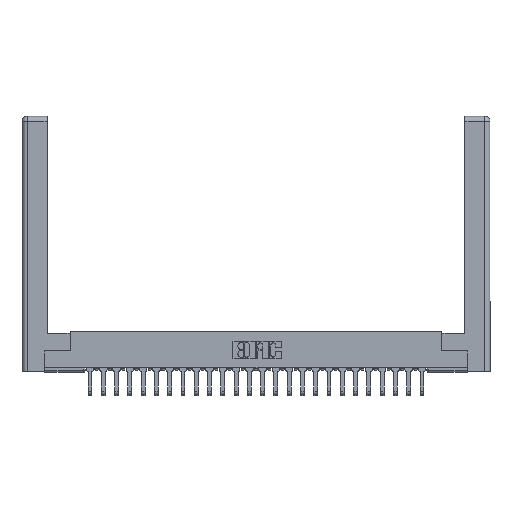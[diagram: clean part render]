
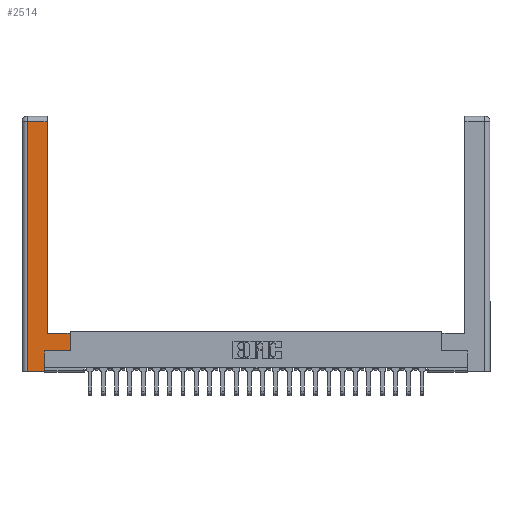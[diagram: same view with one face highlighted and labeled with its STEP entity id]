
A CAD part, top view. The second image highlights one B-rep face of the part: STEP entity #2514.
In plain terms, the highlighted planar face has unit normal (0, 0, 1).
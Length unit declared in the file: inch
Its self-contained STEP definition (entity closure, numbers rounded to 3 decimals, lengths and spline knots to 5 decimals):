
#30 = VECTOR ( 'NONE', #3883, 39.37008 ) ;
#314 = DIRECTION ( 'NONE',  ( -1., 0., 0. ) ) ;
#510 = PLANE ( 'NONE',  #3973 ) ;
#860 = LINE ( 'NONE', #26434, #21745 ) ;
#916 = CARTESIAN_POINT ( 'NONE',  ( 0.565, 0.245, 0. ) ) ;
#1131 = CARTESIAN_POINT ( 'NONE',  ( 0.265, 0.245, 0. ) ) ;
#1563 = CARTESIAN_POINT ( 'NONE',  ( 0.0615, 0., 0. ) ) ;
#1761 = EDGE_CURVE ( 'NONE', #10073, #13633, #22837, .T. ) ;
#2514 = ADVANCED_FACE ( 'NONE', ( #8100 ), #510, .F. ) ;
#2621 = VERTEX_POINT ( 'NONE', #7193 ) ;
#3883 = DIRECTION ( 'NONE',  ( -1., 0., 0. ) ) ;
#3973 = AXIS2_PLACEMENT_3D ( 'NONE', #10960, #25379, #314 ) ;
#4400 = CARTESIAN_POINT ( 'NONE',  ( 0.0615, 0., 0. ) ) ;
#4638 = VERTEX_POINT ( 'NONE', #9826 ) ;
#4655 = VERTEX_POINT ( 'NONE', #23874 ) ;
#4863 = ORIENTED_EDGE ( 'NONE', *, *, #17424, .T. ) ;
#5001 = ORIENTED_EDGE ( 'NONE', *, *, #16443, .T. ) ;
#5208 = DIRECTION ( 'NONE',  ( 0., 1., 0. ) ) ;
#6416 = EDGE_CURVE ( 'NONE', #17836, #2621, #860, .T. ) ;
#7193 = CARTESIAN_POINT ( 'NONE',  ( 0.265, 0., 0. ) ) ;
#7427 = VECTOR ( 'NONE', #21174, 39.37008 ) ;
#7670 = LINE ( 'NONE', #20592, #7977 ) ;
#7977 = VECTOR ( 'NONE', #26803, 39.37008 ) ;
#8100 = FACE_OUTER_BOUND ( 'NONE', #12183, .T. ) ;
#8165 = EDGE_CURVE ( 'NONE', #4655, #4638, #8210, .T. ) ;
#8210 = LINE ( 'NONE', #916, #10479 ) ;
#8674 = CARTESIAN_POINT ( 'NONE',  ( 0.295, 0.45, 0. ) ) ;
#9826 = CARTESIAN_POINT ( 'NONE',  ( 0.565, 0.245, 0. ) ) ;
#10073 = VERTEX_POINT ( 'NONE', #17675 ) ;
#10460 = ORIENTED_EDGE ( 'NONE', *, *, #8165, .T. ) ;
#10479 = VECTOR ( 'NONE', #11371, 39.37008 ) ;
#10960 = CARTESIAN_POINT ( 'NONE',  ( 0., 0., 0. ) ) ;
#11371 = DIRECTION ( 'NONE',  ( 1., 0., 0. ) ) ;
#11389 = ORIENTED_EDGE ( 'NONE', *, *, #15886, .T. ) ;
#11868 = CARTESIAN_POINT ( 'NONE',  ( 0.565, 0.45, 0. ) ) ;
#11870 = VERTEX_POINT ( 'NONE', #26279 ) ;
#12183 = EDGE_LOOP ( 'NONE', ( #4863, #5001, #13068, #23811, #22611, #10460, #11389, #23444 ) ) ;
#12727 = CARTESIAN_POINT ( 'NONE',  ( 0.0615, 2.94, 0. ) ) ;
#13068 = ORIENTED_EDGE ( 'NONE', *, *, #19229, .T. ) ;
#13633 = VERTEX_POINT ( 'NONE', #8674 ) ;
#13782 = LINE ( 'NONE', #1131, #24239 ) ;
#15236 = LINE ( 'NONE', #4400, #7427 ) ;
#15886 = EDGE_CURVE ( 'NONE', #4638, #10073, #22467, .T. ) ;
#16443 = EDGE_CURVE ( 'NONE', #24471, #11870, #17526, .T. ) ;
#17231 = VECTOR ( 'NONE', #26455, 39.37008 ) ;
#17424 = EDGE_CURVE ( 'NONE', #13633, #24471, #7670, .T. ) ;
#17526 = LINE ( 'NONE', #12727, #23720 ) ;
#17675 = CARTESIAN_POINT ( 'NONE',  ( 0.565, 0.45, 0. ) ) ;
#17836 = VERTEX_POINT ( 'NONE', #1563 ) ;
#18246 = CARTESIAN_POINT ( 'NONE',  ( 0.295, 2.94, 0. ) ) ;
#18678 = CARTESIAN_POINT ( 'NONE',  ( 0.295, 0.45, 0. ) ) ;
#19229 = EDGE_CURVE ( 'NONE', #11870, #17836, #15236, .T. ) ;
#20037 = DIRECTION ( 'NONE',  ( 1., 0., 0. ) ) ;
#20592 = CARTESIAN_POINT ( 'NONE',  ( 0.295, 3., 0. ) ) ;
#21174 = DIRECTION ( 'NONE',  ( 0., -1., 0. ) ) ;
#21584 = DIRECTION ( 'NONE',  ( -1., 0., 0. ) ) ;
#21745 = VECTOR ( 'NONE', #20037, 39.37008 ) ;
#22467 = LINE ( 'NONE', #11868, #17231 ) ;
#22541 = EDGE_CURVE ( 'NONE', #2621, #4655, #13782, .T. ) ;
#22611 = ORIENTED_EDGE ( 'NONE', *, *, #22541, .T. ) ;
#22837 = LINE ( 'NONE', #18678, #30 ) ;
#23444 = ORIENTED_EDGE ( 'NONE', *, *, #1761, .T. ) ;
#23720 = VECTOR ( 'NONE', #21584, 39.37008 ) ;
#23811 = ORIENTED_EDGE ( 'NONE', *, *, #6416, .T. ) ;
#23874 = CARTESIAN_POINT ( 'NONE',  ( 0.265, 0.245, 0. ) ) ;
#24239 = VECTOR ( 'NONE', #5208, 39.37008 ) ;
#24471 = VERTEX_POINT ( 'NONE', #18246 ) ;
#25379 = DIRECTION ( 'NONE',  ( 0., 0., -1. ) ) ;
#26279 = CARTESIAN_POINT ( 'NONE',  ( 0.0615, 2.94, 0. ) ) ;
#26434 = CARTESIAN_POINT ( 'NONE',  ( 0.265, 0., 0. ) ) ;
#26455 = DIRECTION ( 'NONE',  ( 0., 1., 0. ) ) ;
#26803 = DIRECTION ( 'NONE',  ( 0., 1., 0. ) ) ;
